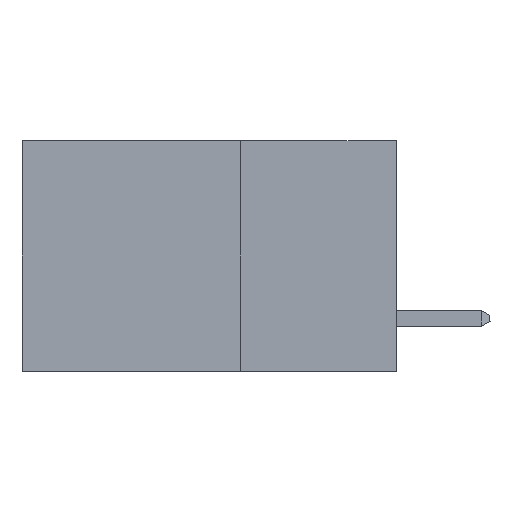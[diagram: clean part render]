
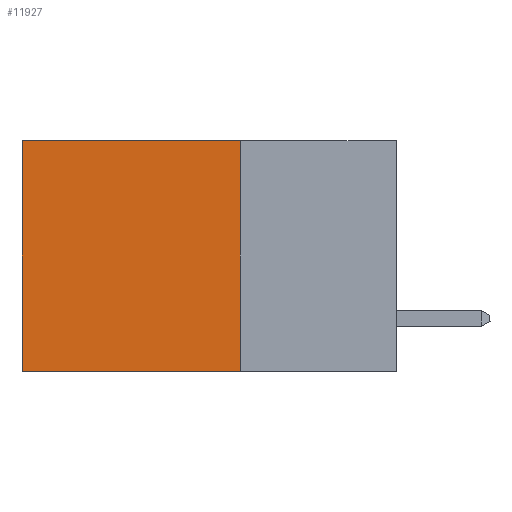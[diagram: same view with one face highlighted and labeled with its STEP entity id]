
A CAD part, left-side view. The second image highlights one B-rep face of the part: STEP entity #11927.
In plain terms, the highlighted planar face has unit normal (-1, 0, 0).
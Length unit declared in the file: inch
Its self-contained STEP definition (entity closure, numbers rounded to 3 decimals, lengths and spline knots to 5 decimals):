
#1508 = EDGE_CURVE ( 'NONE', #18455, #19745, #24393, .T. ) ;
#1597 = EDGE_CURVE ( 'NONE', #4609, #18455, #5176, .T. ) ;
#1671 = CARTESIAN_POINT ( 'NONE',  ( 0.298, 0.6, 0. ) ) ;
#2681 = FACE_OUTER_BOUND ( 'NONE', #10908, .T. ) ;
#4606 = LINE ( 'NONE', #15319, #9366 ) ;
#4609 = VERTEX_POINT ( 'NONE', #8436 ) ;
#4666 = DIRECTION ( 'NONE',  ( 1., 0., 0. ) ) ;
#4764 = CARTESIAN_POINT ( 'NONE',  ( 0.298, 0.6, 0. ) ) ;
#5045 = CARTESIAN_POINT ( 'NONE',  ( 0.298, 0.25, -0.37 ) ) ;
#5176 = LINE ( 'NONE', #13538, #25951 ) ;
#5608 = EDGE_CURVE ( 'NONE', #4609, #20229, #4606, .T. ) ;
#7729 = VECTOR ( 'NONE', #14789, 39.37008 ) ;
#8436 = CARTESIAN_POINT ( 'NONE',  ( 0.298, 0.25, 0. ) ) ;
#8980 = DIRECTION ( 'NONE',  ( 0., 0., -1. ) ) ;
#9353 = LINE ( 'NONE', #4764, #9992 ) ;
#9366 = VECTOR ( 'NONE', #23401, 39.37008 ) ;
#9992 = VECTOR ( 'NONE', #12838, 39.37008 ) ;
#10303 = ORIENTED_EDGE ( 'NONE', *, *, #24954, .T. ) ;
#10699 = CARTESIAN_POINT ( 'NONE',  ( 0.298, 0.25, 0. ) ) ;
#10908 = EDGE_LOOP ( 'NONE', ( #10303, #11434, #22693, #21836 ) ) ;
#11434 = ORIENTED_EDGE ( 'NONE', *, *, #1508, .F. ) ;
#11927 = ADVANCED_FACE ( 'NONE', ( #2681 ), #16781, .F. ) ;
#12838 = DIRECTION ( 'NONE',  ( 0., 0., -1. ) ) ;
#13538 = CARTESIAN_POINT ( 'NONE',  ( 0.298, 0.25, 0. ) ) ;
#14789 = DIRECTION ( 'NONE',  ( 0., 1., 0. ) ) ;
#15319 = CARTESIAN_POINT ( 'NONE',  ( 0.298, 0.25, 0. ) ) ;
#15600 = CARTESIAN_POINT ( 'NONE',  ( 0.298, 0.6, -0.37 ) ) ;
#16781 = PLANE ( 'NONE',  #21512 ) ;
#18455 = VERTEX_POINT ( 'NONE', #24991 ) ;
#18798 = DIRECTION ( 'NONE',  ( 0., 0., -1. ) ) ;
#19745 = VERTEX_POINT ( 'NONE', #15600 ) ;
#20229 = VERTEX_POINT ( 'NONE', #1671 ) ;
#21512 = AXIS2_PLACEMENT_3D ( 'NONE', #10699, #4666, #18798 ) ;
#21836 = ORIENTED_EDGE ( 'NONE', *, *, #5608, .T. ) ;
#22693 = ORIENTED_EDGE ( 'NONE', *, *, #1597, .F. ) ;
#23401 = DIRECTION ( 'NONE',  ( 0., 1., 0. ) ) ;
#24393 = LINE ( 'NONE', #5045, #7729 ) ;
#24954 = EDGE_CURVE ( 'NONE', #20229, #19745, #9353, .T. ) ;
#24991 = CARTESIAN_POINT ( 'NONE',  ( 0.298, 0.25, -0.37 ) ) ;
#25951 = VECTOR ( 'NONE', #8980, 39.37008 ) ;
